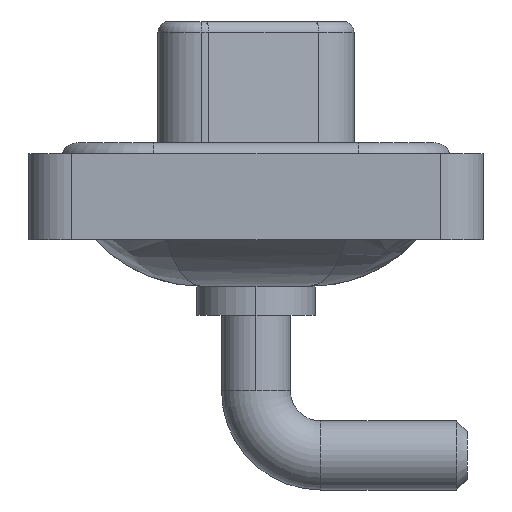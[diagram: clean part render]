
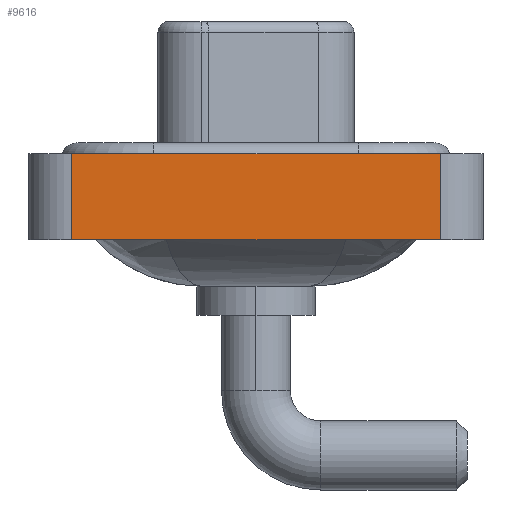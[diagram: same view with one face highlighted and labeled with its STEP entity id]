
A CAD part, left-side view. The second image highlights one B-rep face of the part: STEP entity #9616.
In plain terms, the highlighted planar face has unit normal (-1, 0, 0).
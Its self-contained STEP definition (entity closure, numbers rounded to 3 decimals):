
#82 = LINE ( 'NONE', #15211, #4326 ) ;
#853 = VERTEX_POINT ( 'NONE', #1547 ) ;
#1073 = VECTOR ( 'NONE', #5665, 1000. ) ;
#1547 = CARTESIAN_POINT ( 'NONE',  ( -7.35, -8.55, 0.4 ) ) ;
#1636 = LINE ( 'NONE', #16949, #1073 ) ;
#1747 = CARTESIAN_POINT ( 'NONE',  ( -7.35, 8.55, -3.6 ) ) ;
#3674 = CARTESIAN_POINT ( 'NONE',  ( -7.35, -8.55, 0.4 ) ) ;
#4326 = VECTOR ( 'NONE', #8229, 1000. ) ;
#5212 = EDGE_CURVE ( 'NONE', #17094, #14764, #16636, .T. ) ;
#5665 = DIRECTION ( 'NONE',  ( 0., 0., 1. ) ) ;
#6620 = PLANE ( 'NONE',  #10955 ) ;
#6678 = EDGE_CURVE ( 'NONE', #14764, #853, #8054, .T. ) ;
#7001 = ORIENTED_EDGE ( 'NONE', *, *, #11530, .T. ) ;
#7985 = DIRECTION ( 'NONE',  ( -1., 0., 0. ) ) ;
#8054 = LINE ( 'NONE', #3674, #15747 ) ;
#8118 = ORIENTED_EDGE ( 'NONE', *, *, #5212, .F. ) ;
#8229 = DIRECTION ( 'NONE',  ( 0., -1., 0. ) ) ;
#8453 = CARTESIAN_POINT ( 'NONE',  ( -7.35, -8.55, -3.6 ) ) ;
#9162 = CARTESIAN_POINT ( 'NONE',  ( -7.35, -8.55, -3.6 ) ) ;
#9616 = ADVANCED_FACE ( 'NONE', ( #17718 ), #6620, .T. ) ;
#9646 = CARTESIAN_POINT ( 'NONE',  ( -7.35, 8.55, -3.6 ) ) ;
#10428 = VERTEX_POINT ( 'NONE', #8453 ) ;
#10526 = CARTESIAN_POINT ( 'NONE',  ( -7.35, 8.55, 0.4 ) ) ;
#10955 = AXIS2_PLACEMENT_3D ( 'NONE', #9162, #7985, #13208 ) ;
#11530 = EDGE_CURVE ( 'NONE', #17094, #10428, #82, .T. ) ;
#11702 = ORIENTED_EDGE ( 'NONE', *, *, #17512, .T. ) ;
#11958 = EDGE_LOOP ( 'NONE', ( #11702, #16228, #8118, #7001 ) ) ;
#12479 = VECTOR ( 'NONE', #18105, 1000. ) ;
#13208 = DIRECTION ( 'NONE',  ( 0., 0., 1. ) ) ;
#14764 = VERTEX_POINT ( 'NONE', #10526 ) ;
#14933 = DIRECTION ( 'NONE',  ( 0., -1., 0. ) ) ;
#15211 = CARTESIAN_POINT ( 'NONE',  ( -7.35, -8.55, -3.6 ) ) ;
#15747 = VECTOR ( 'NONE', #14933, 1000. ) ;
#16228 = ORIENTED_EDGE ( 'NONE', *, *, #6678, .F. ) ;
#16636 = LINE ( 'NONE', #9646, #12479 ) ;
#16949 = CARTESIAN_POINT ( 'NONE',  ( -7.35, -8.55, -3.6 ) ) ;
#17094 = VERTEX_POINT ( 'NONE', #1747 ) ;
#17512 = EDGE_CURVE ( 'NONE', #10428, #853, #1636, .T. ) ;
#17718 = FACE_OUTER_BOUND ( 'NONE', #11958, .T. ) ;
#18105 = DIRECTION ( 'NONE',  ( 0., 0., 1. ) ) ;
